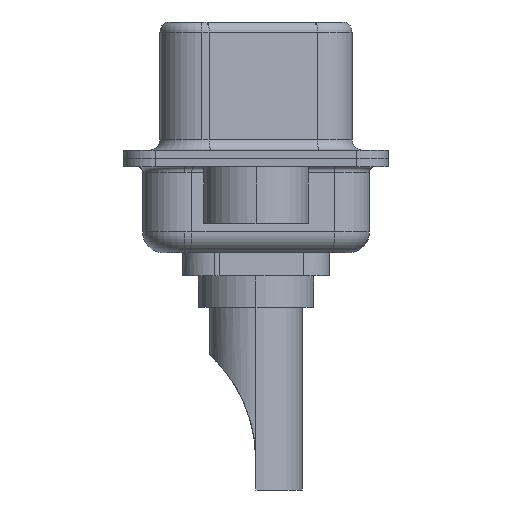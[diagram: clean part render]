
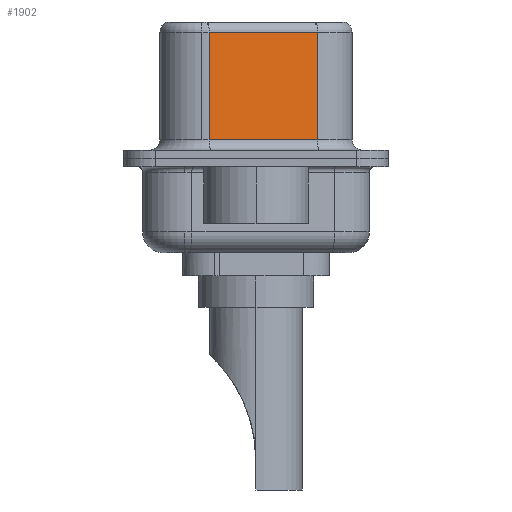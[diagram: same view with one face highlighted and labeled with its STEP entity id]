
A CAD part, left-side view. The second image highlights one B-rep face of the part: STEP entity #1902.
In plain terms, the highlighted planar face has unit normal (-0.985, -0.174, 0).
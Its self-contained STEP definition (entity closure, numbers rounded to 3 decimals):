
#217 = VERTEX_POINT ( 'NONE', #18183 ) ;
#934 = CARTESIAN_POINT ( 'NONE',  ( 4.58, -2.927, 0.9 ) ) ;
#1136 = EDGE_CURVE ( 'NONE', #217, #5157, #8555, .T. ) ;
#1213 = FACE_OUTER_BOUND ( 'NONE', #1431, .T. ) ;
#1431 = EDGE_LOOP ( 'NONE', ( #7313, #14606, #2998, #7214 ) ) ;
#1902 = ADVANCED_FACE ( 'NONE', ( #1213 ), #10067, .F. ) ;
#2319 = VECTOR ( 'NONE', #5877, 1000. ) ;
#2565 = CARTESIAN_POINT ( 'NONE',  ( 3.67, 2.233, 0.9 ) ) ;
#2998 = ORIENTED_EDGE ( 'NONE', *, *, #17033, .T. ) ;
#3087 = EDGE_CURVE ( 'NONE', #3308, #18559, #16978, .T. ) ;
#3308 = VERTEX_POINT ( 'NONE', #2565 ) ;
#4396 = CARTESIAN_POINT ( 'NONE',  ( 3.67, 2.233, 6.02 ) ) ;
#4711 = DIRECTION ( 'NONE',  ( -0.174, 0.985, 0. ) ) ;
#5028 = VECTOR ( 'NONE', #11483, 1000. ) ;
#5157 = VERTEX_POINT ( 'NONE', #4396 ) ;
#5354 = VECTOR ( 'NONE', #4711, 1000. ) ;
#5497 = LINE ( 'NONE', #18915, #5028 ) ;
#5877 = DIRECTION ( 'NONE',  ( 0., 0., -1. ) ) ;
#6037 = DIRECTION ( 'NONE',  ( 0.174, -0.985, 0. ) ) ;
#6118 = DIRECTION ( 'NONE',  ( 0.985, 0.174, 0. ) ) ;
#7214 = ORIENTED_EDGE ( 'NONE', *, *, #3087, .T. ) ;
#7313 = ORIENTED_EDGE ( 'NONE', *, *, #8144, .F. ) ;
#8144 = EDGE_CURVE ( 'NONE', #217, #18559, #5497, .T. ) ;
#8555 = LINE ( 'NONE', #9073, #5354 ) ;
#9073 = CARTESIAN_POINT ( 'NONE',  ( 4.58, -2.927, 6.02 ) ) ;
#10067 = PLANE ( 'NONE',  #14889 ) ;
#10076 = LINE ( 'NONE', #18872, #2319 ) ;
#10344 = DIRECTION ( 'NONE',  ( -0.174, 0.985, 0. ) ) ;
#11483 = DIRECTION ( 'NONE',  ( 0., 0., -1. ) ) ;
#14171 = CARTESIAN_POINT ( 'NONE',  ( 4.58, -2.927, 6.52 ) ) ;
#14606 = ORIENTED_EDGE ( 'NONE', *, *, #1136, .T. ) ;
#14739 = CARTESIAN_POINT ( 'NONE',  ( 4.58, -2.927, 0.9 ) ) ;
#14889 = AXIS2_PLACEMENT_3D ( 'NONE', #14171, #6118, #10344 ) ;
#16516 = VECTOR ( 'NONE', #6037, 1000. ) ;
#16978 = LINE ( 'NONE', #14739, #16516 ) ;
#17033 = EDGE_CURVE ( 'NONE', #5157, #3308, #10076, .T. ) ;
#18183 = CARTESIAN_POINT ( 'NONE',  ( 4.58, -2.927, 6.02 ) ) ;
#18559 = VERTEX_POINT ( 'NONE', #934 ) ;
#18872 = CARTESIAN_POINT ( 'NONE',  ( 3.67, 2.233, 6.52 ) ) ;
#18915 = CARTESIAN_POINT ( 'NONE',  ( 4.58, -2.927, 6.52 ) ) ;
